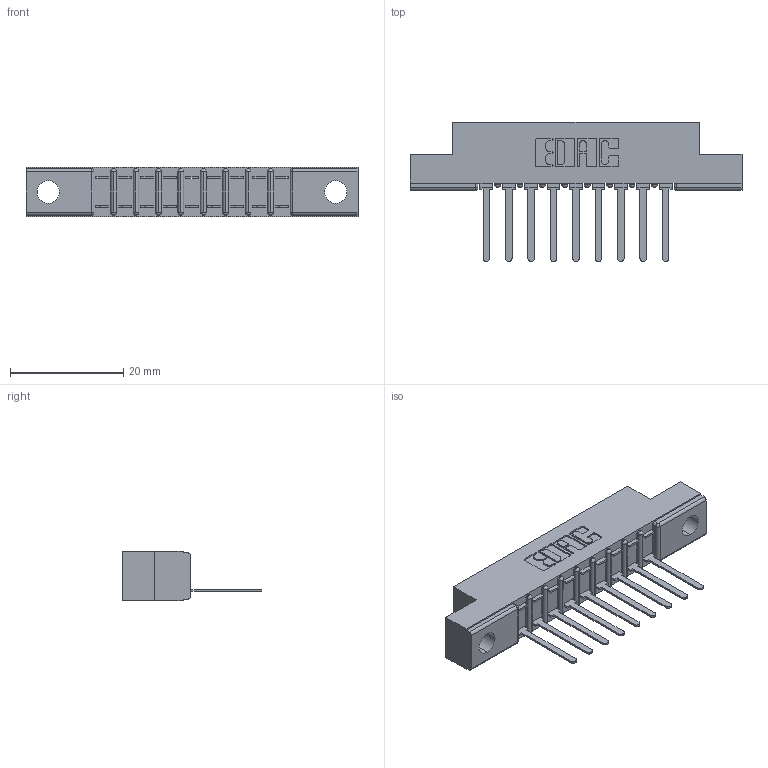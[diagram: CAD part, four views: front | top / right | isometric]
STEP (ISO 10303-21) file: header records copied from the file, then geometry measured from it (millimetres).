
FILE_DESCRIPTION (( 'STEP AP203' ), '1' );
FILE_NAME ('357-009-541-104.STEP', '2019-09-16T18:03:57', ( '' ), ( '' ), 'SwSTEP 2.0', 'SolidWorks 2016', '' );
FILE_SCHEMA (( 'CONFIG_CONTROL_DESIGN' ));
Length unit declared in the file: inch
Products named in the file (3): 357-009-541-104; 307-290-002_541; 307 Part_.156 Dia Mounting Holes
Assembly tree (10 placements, depth 2):
  357-009-541-104
    307 Part_.156 Dia Mounting Holes
    307-290-002_541  x9
Bounding box: 58.67 x 24.59 x 8.71 mm (x, y, z)
Volume: 3786.2 mm3; surface area: 6207.7 mm2
Topology: 10 solids, 10 shells, 808 faces, 2447 edges, 1602 vertices
Faces by surface type: plane 489, cylinder 299, sphere 20
Entity records: 12920 total; most frequent: CARTESIAN_POINT 2178, ORIENTED_EDGE 2166, DIRECTION 2123, EDGE_CURVE 1083, VECTOR 821, LINE 821, VERTEX_POINT 706, AXIS2_PLACEMENT_3D 651
